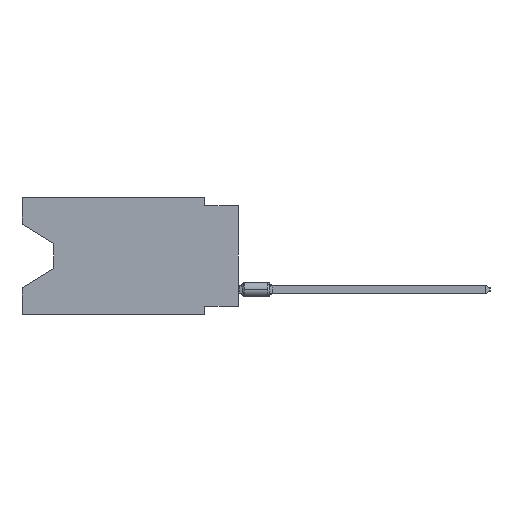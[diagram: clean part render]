
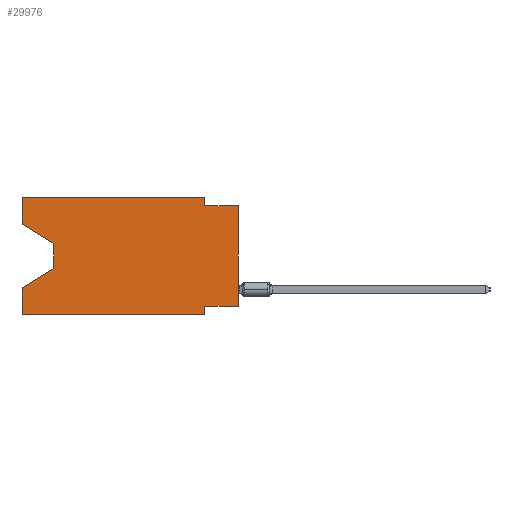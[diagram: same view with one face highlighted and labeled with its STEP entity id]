
A CAD part, left-side view. The second image highlights one B-rep face of the part: STEP entity #29976.
In plain terms, the highlighted planar face has unit normal (-1, 0, 0).
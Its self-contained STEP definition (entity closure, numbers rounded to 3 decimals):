
#141 = CARTESIAN_POINT ( 'NONE',  ( 0., 13.97, -5.385 ) ) ;
#1084 = EDGE_CURVE ( 'NONE', #6473, #16849, #20135, .T. ) ;
#1313 = VECTOR ( 'NONE', #10881, 1000. ) ;
#1587 = CARTESIAN_POINT ( 'NONE',  ( 0., 13.97, -5.385 ) ) ;
#1644 = CARTESIAN_POINT ( 'NONE',  ( 0., 16.383, 0. ) ) ;
#1949 = EDGE_CURVE ( 'NONE', #18259, #13770, #21244, .T. ) ;
#1959 = CARTESIAN_POINT ( 'NONE',  ( 0., 2.54, 0. ) ) ;
#2231 = VERTEX_POINT ( 'NONE', #20297 ) ;
#2707 = VERTEX_POINT ( 'NONE', #1959 ) ;
#3023 = VECTOR ( 'NONE', #30162, 1000. ) ;
#3107 = EDGE_CURVE ( 'NONE', #23205, #18259, #23145, .T. ) ;
#3472 = LINE ( 'NONE', #21998, #1313 ) ;
#4251 = ORIENTED_EDGE ( 'NONE', *, *, #25701, .T. ) ;
#4424 = DIRECTION ( 'NONE',  ( 0., 0., -1. ) ) ;
#4459 = VECTOR ( 'NONE', #22292, 1000. ) ;
#4645 = ORIENTED_EDGE ( 'NONE', *, *, #8114, .T. ) ;
#5279 = DIRECTION ( 'NONE',  ( 0., 0., -1. ) ) ;
#5919 = LINE ( 'NONE', #17649, #21693 ) ;
#6473 = VERTEX_POINT ( 'NONE', #12445 ) ;
#7079 = DIRECTION ( 'NONE',  ( 0., 0.855, -0.519 ) ) ;
#7597 = CARTESIAN_POINT ( 'NONE',  ( 0., 16.383, 0. ) ) ;
#7635 = CARTESIAN_POINT ( 'NONE',  ( 0., 0., 0. ) ) ;
#7746 = FACE_OUTER_BOUND ( 'NONE', #23897, .T. ) ;
#8114 = EDGE_CURVE ( 'NONE', #18455, #16849, #5919, .T. ) ;
#8926 = DIRECTION ( 'NONE',  ( 0., -1., 0. ) ) ;
#9089 = EDGE_CURVE ( 'NONE', #26273, #21739, #15579, .T. ) ;
#9258 = CARTESIAN_POINT ( 'NONE',  ( 0., 16.383, -2.038 ) ) ;
#9552 = LINE ( 'NONE', #14340, #27415 ) ;
#9985 = ORIENTED_EDGE ( 'NONE', *, *, #10402, .T. ) ;
#10402 = EDGE_CURVE ( 'NONE', #13770, #27837, #18956, .T. ) ;
#10662 = VECTOR ( 'NONE', #26109, 1000. ) ;
#10881 = DIRECTION ( 'NONE',  ( 0., 0., 1. ) ) ;
#11863 = CARTESIAN_POINT ( 'NONE',  ( 0., 2.54, -8.89 ) ) ;
#11876 = VECTOR ( 'NONE', #8926, 1000. ) ;
#11903 = CARTESIAN_POINT ( 'NONE',  ( 0., 2.54, -0.635 ) ) ;
#12445 = CARTESIAN_POINT ( 'NONE',  ( 0., 2.54, -8.255 ) ) ;
#12682 = EDGE_CURVE ( 'NONE', #14537, #6473, #9552, .T. ) ;
#13048 = ORIENTED_EDGE ( 'NONE', *, *, #24902, .F. ) ;
#13162 = ORIENTED_EDGE ( 'NONE', *, *, #12682, .F. ) ;
#13609 = CARTESIAN_POINT ( 'NONE',  ( 0., 16.383, -2.038 ) ) ;
#13705 = DIRECTION ( 'NONE',  ( 0., 0., 1. ) ) ;
#13749 = CARTESIAN_POINT ( 'NONE',  ( 0., 13.97, -3.505 ) ) ;
#13770 = VERTEX_POINT ( 'NONE', #1587 ) ;
#13855 = CARTESIAN_POINT ( 'NONE',  ( 0., 16.383, -6.852 ) ) ;
#14340 = CARTESIAN_POINT ( 'NONE',  ( 0., 0., -8.255 ) ) ;
#14537 = VERTEX_POINT ( 'NONE', #29642 ) ;
#15066 = ORIENTED_EDGE ( 'NONE', *, *, #1949, .T. ) ;
#15579 = LINE ( 'NONE', #23105, #11876 ) ;
#15704 = ORIENTED_EDGE ( 'NONE', *, *, #27167, .F. ) ;
#16849 = VERTEX_POINT ( 'NONE', #11863 ) ;
#16857 = PLANE ( 'NONE',  #21655 ) ;
#17166 = DIRECTION ( 'NONE',  ( 1., 0., 0. ) ) ;
#17527 = CARTESIAN_POINT ( 'NONE',  ( 0., 2.54, -8.89 ) ) ;
#17649 = CARTESIAN_POINT ( 'NONE',  ( 0., 16.383, -8.89 ) ) ;
#18259 = VERTEX_POINT ( 'NONE', #13749 ) ;
#18455 = VERTEX_POINT ( 'NONE', #19589 ) ;
#18956 = LINE ( 'NONE', #141, #27694 ) ;
#19195 = VECTOR ( 'NONE', #13705, 1000. ) ;
#19589 = CARTESIAN_POINT ( 'NONE',  ( 0., 16.383, -8.89 ) ) ;
#19955 = DIRECTION ( 'NONE',  ( 0., -1., 0. ) ) ;
#19998 = ORIENTED_EDGE ( 'NONE', *, *, #20397, .F. ) ;
#20135 = LINE ( 'NONE', #17527, #22796 ) ;
#20297 = CARTESIAN_POINT ( 'NONE',  ( 0., 16.383, 0. ) ) ;
#20397 = EDGE_CURVE ( 'NONE', #23205, #2231, #3472, .T. ) ;
#20864 = VECTOR ( 'NONE', #30237, 1000. ) ;
#21244 = LINE ( 'NONE', #23702, #30178 ) ;
#21655 = AXIS2_PLACEMENT_3D ( 'NONE', #7597, #17166, #5279 ) ;
#21693 = VECTOR ( 'NONE', #19955, 1000. ) ;
#21739 = VERTEX_POINT ( 'NONE', #27825 ) ;
#21998 = CARTESIAN_POINT ( 'NONE',  ( 0., 16.383, 0. ) ) ;
#22220 = LINE ( 'NONE', #24676, #19195 ) ;
#22292 = DIRECTION ( 'NONE',  ( 0., 0., 1. ) ) ;
#22607 = DIRECTION ( 'NONE',  ( 0., 0., -1. ) ) ;
#22796 = VECTOR ( 'NONE', #22607, 1000. ) ;
#23105 = CARTESIAN_POINT ( 'NONE',  ( 0., 0., -0.635 ) ) ;
#23145 = LINE ( 'NONE', #9258, #20864 ) ;
#23188 = CARTESIAN_POINT ( 'NONE',  ( 0., 2.54, 0. ) ) ;
#23205 = VERTEX_POINT ( 'NONE', #13609 ) ;
#23702 = CARTESIAN_POINT ( 'NONE',  ( 0., 13.97, -3.505 ) ) ;
#23703 = ORIENTED_EDGE ( 'NONE', *, *, #1084, .F. ) ;
#23737 = DIRECTION ( 'NONE',  ( 0., 1., 0. ) ) ;
#23897 = EDGE_LOOP ( 'NONE', ( #30101, #15066, #9985, #13048, #4645, #23703, #13162, #4251, #27042, #15704, #29101, #19998 ) ) ;
#24676 = CARTESIAN_POINT ( 'NONE',  ( 0., 16.383, 0. ) ) ;
#24902 = EDGE_CURVE ( 'NONE', #18455, #27837, #22220, .T. ) ;
#25085 = LINE ( 'NONE', #1644, #3023 ) ;
#25701 = EDGE_CURVE ( 'NONE', #14537, #21739, #29231, .T. ) ;
#25802 = LINE ( 'NONE', #23188, #10662 ) ;
#26109 = DIRECTION ( 'NONE',  ( 0., 0., -1. ) ) ;
#26273 = VERTEX_POINT ( 'NONE', #11903 ) ;
#26646 = EDGE_CURVE ( 'NONE', #2231, #2707, #25085, .T. ) ;
#27042 = ORIENTED_EDGE ( 'NONE', *, *, #9089, .F. ) ;
#27167 = EDGE_CURVE ( 'NONE', #2707, #26273, #25802, .T. ) ;
#27415 = VECTOR ( 'NONE', #23737, 1000. ) ;
#27694 = VECTOR ( 'NONE', #7079, 1000. ) ;
#27825 = CARTESIAN_POINT ( 'NONE',  ( 0., 0., -0.635 ) ) ;
#27837 = VERTEX_POINT ( 'NONE', #13855 ) ;
#29101 = ORIENTED_EDGE ( 'NONE', *, *, #26646, .F. ) ;
#29231 = LINE ( 'NONE', #7635, #4459 ) ;
#29642 = CARTESIAN_POINT ( 'NONE',  ( 0., 0., -8.255 ) ) ;
#29976 = ADVANCED_FACE ( 'NONE', ( #7746 ), #16857, .F. ) ;
#30101 = ORIENTED_EDGE ( 'NONE', *, *, #3107, .T. ) ;
#30162 = DIRECTION ( 'NONE',  ( 0., -1., 0. ) ) ;
#30178 = VECTOR ( 'NONE', #4424, 1000. ) ;
#30237 = DIRECTION ( 'NONE',  ( 0., -0.855, -0.519 ) ) ;
